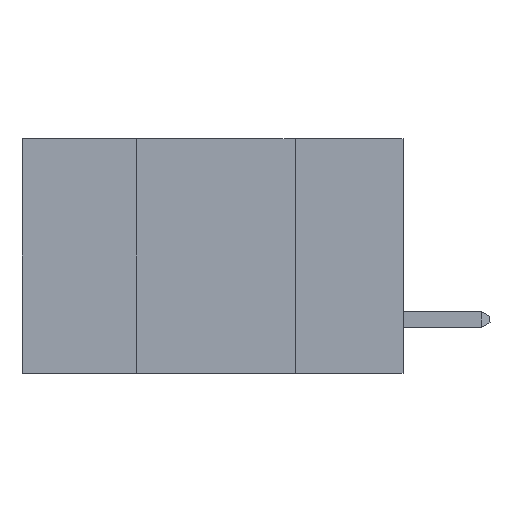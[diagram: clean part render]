
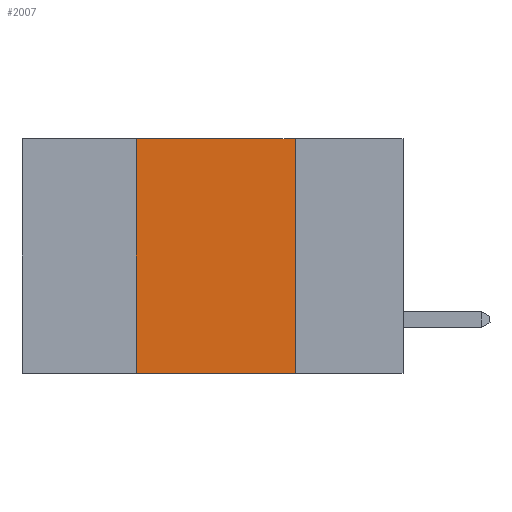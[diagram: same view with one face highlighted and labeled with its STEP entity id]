
A CAD part, left-side view. The second image highlights one B-rep face of the part: STEP entity #2007.
In plain terms, the highlighted planar face has unit normal (-1, 0, 0).
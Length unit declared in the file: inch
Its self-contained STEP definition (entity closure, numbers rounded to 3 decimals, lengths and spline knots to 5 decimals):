
#102 = LINE ( 'NONE', #7719, #11655 ) ;
#1054 = CARTESIAN_POINT ( 'NONE',  ( 0., 0.42, -0.37 ) ) ;
#1588 = DIRECTION ( 'NONE',  ( 0., -1., 0. ) ) ;
#2007 = ADVANCED_FACE ( 'NONE', ( #5160 ), #6596, .F. ) ;
#2907 = EDGE_LOOP ( 'NONE', ( #9819, #17971, #17100, #13841 ) ) ;
#3221 = VERTEX_POINT ( 'NONE', #15116 ) ;
#3620 = LINE ( 'NONE', #4546, #7667 ) ;
#3697 = DIRECTION ( 'NONE',  ( 1., 0., 0. ) ) ;
#4546 = CARTESIAN_POINT ( 'NONE',  ( 0., 0.6, 0. ) ) ;
#5160 = FACE_OUTER_BOUND ( 'NONE', #2907, .T. ) ;
#5391 = VECTOR ( 'NONE', #7646, 39.37008 ) ;
#6056 = VERTEX_POINT ( 'NONE', #1054 ) ;
#6083 = LINE ( 'NONE', #17292, #9639 ) ;
#6398 = DIRECTION ( 'NONE',  ( 0., 0., -1. ) ) ;
#6596 = PLANE ( 'NONE',  #16187 ) ;
#7646 = DIRECTION ( 'NONE',  ( 0., -1., 0. ) ) ;
#7667 = VECTOR ( 'NONE', #1588, 39.37008 ) ;
#7719 = CARTESIAN_POINT ( 'NONE',  ( 0., 0.42, 0. ) ) ;
#7842 = CARTESIAN_POINT ( 'NONE',  ( 0., 0.17, 0. ) ) ;
#8842 = EDGE_CURVE ( 'NONE', #18712, #17224, #3620, .T. ) ;
#9223 = DIRECTION ( 'NONE',  ( 0., 0., 1. ) ) ;
#9639 = VECTOR ( 'NONE', #14298, 39.37008 ) ;
#9819 = ORIENTED_EDGE ( 'NONE', *, *, #13142, .F. ) ;
#10633 = CARTESIAN_POINT ( 'NONE',  ( 0., 0.6, -0.37 ) ) ;
#11655 = VECTOR ( 'NONE', #9223, 39.37008 ) ;
#12638 = CARTESIAN_POINT ( 'NONE',  ( 0., 0.42, 0. ) ) ;
#13142 = EDGE_CURVE ( 'NONE', #17224, #3221, #6083, .T. ) ;
#13841 = ORIENTED_EDGE ( 'NONE', *, *, #19114, .T. ) ;
#14298 = DIRECTION ( 'NONE',  ( 0., 0., -1. ) ) ;
#15116 = CARTESIAN_POINT ( 'NONE',  ( 0., 0.17, -0.37 ) ) ;
#16161 = EDGE_CURVE ( 'NONE', #6056, #18712, #102, .T. ) ;
#16187 = AXIS2_PLACEMENT_3D ( 'NONE', #16780, #3697, #6398 ) ;
#16780 = CARTESIAN_POINT ( 'NONE',  ( 0., 0.6, 0. ) ) ;
#17100 = ORIENTED_EDGE ( 'NONE', *, *, #16161, .F. ) ;
#17224 = VERTEX_POINT ( 'NONE', #7842 ) ;
#17292 = CARTESIAN_POINT ( 'NONE',  ( 0., 0.17, 0. ) ) ;
#17366 = LINE ( 'NONE', #10633, #5391 ) ;
#17971 = ORIENTED_EDGE ( 'NONE', *, *, #8842, .F. ) ;
#18712 = VERTEX_POINT ( 'NONE', #12638 ) ;
#19114 = EDGE_CURVE ( 'NONE', #6056, #3221, #17366, .T. ) ;
